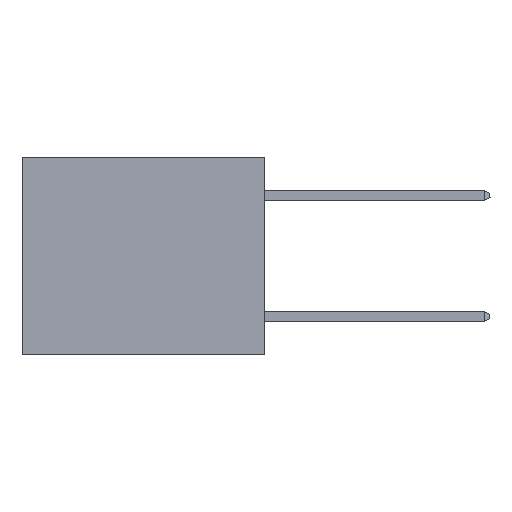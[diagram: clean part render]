
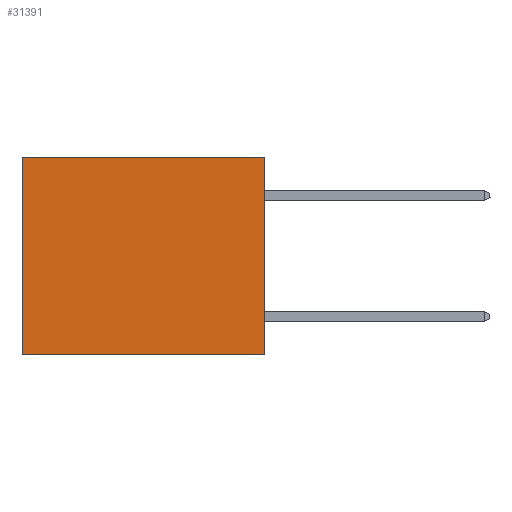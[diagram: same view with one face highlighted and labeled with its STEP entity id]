
A CAD part, left-side view. The second image highlights one B-rep face of the part: STEP entity #31391.
In plain terms, the highlighted planar face has unit normal (-1, 0, 0).
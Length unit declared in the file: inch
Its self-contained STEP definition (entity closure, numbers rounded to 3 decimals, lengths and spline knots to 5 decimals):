
#1313 = LINE ( 'NONE', #6513, #23209 ) ;
#1615 = CARTESIAN_POINT ( 'NONE',  ( 0.3165, 0., -0.49 ) ) ;
#2115 = VERTEX_POINT ( 'NONE', #4589 ) ;
#3891 = ORIENTED_EDGE ( 'NONE', *, *, #5600, .F. ) ;
#4589 = CARTESIAN_POINT ( 'NONE',  ( 0.3165, 0.6, -0.49 ) ) ;
#4840 = EDGE_CURVE ( 'NONE', #29990, #2115, #23736, .T. ) ;
#5600 = EDGE_CURVE ( 'NONE', #15336, #2115, #1313, .T. ) ;
#6211 = DIRECTION ( 'NONE',  ( 0., 0., -1. ) ) ;
#6513 = CARTESIAN_POINT ( 'NONE',  ( 0.3165, 0., -0.49 ) ) ;
#8100 = FACE_OUTER_BOUND ( 'NONE', #31396, .T. ) ;
#8505 = LINE ( 'NONE', #28277, #10466 ) ;
#9212 = DIRECTION ( 'NONE',  ( 0., 1., 0. ) ) ;
#10284 = CARTESIAN_POINT ( 'NONE',  ( 0.3165, 0.6, -0.49 ) ) ;
#10466 = VECTOR ( 'NONE', #6211, 39.37008 ) ;
#10554 = VERTEX_POINT ( 'NONE', #13861 ) ;
#11129 = EDGE_CURVE ( 'NONE', #10554, #29990, #11535, .T. ) ;
#11535 = LINE ( 'NONE', #16831, #26160 ) ;
#12883 = DIRECTION ( 'NONE',  ( 0., 0., -1. ) ) ;
#12912 = ORIENTED_EDGE ( 'NONE', *, *, #11129, .T. ) ;
#13569 = ORIENTED_EDGE ( 'NONE', *, *, #18729, .F. ) ;
#13861 = CARTESIAN_POINT ( 'NONE',  ( 0.3165, 0., 0. ) ) ;
#15336 = VERTEX_POINT ( 'NONE', #22647 ) ;
#16187 = DIRECTION ( 'NONE',  ( 1., 0., 0. ) ) ;
#16831 = CARTESIAN_POINT ( 'NONE',  ( 0.3165, 0., 0. ) ) ;
#18729 = EDGE_CURVE ( 'NONE', #10554, #15336, #8505, .T. ) ;
#19314 = DIRECTION ( 'NONE',  ( 0., 1., 0. ) ) ;
#21388 = VECTOR ( 'NONE', #12883, 39.37008 ) ;
#21995 = CARTESIAN_POINT ( 'NONE',  ( 0.3165, 0.6, 0. ) ) ;
#22647 = CARTESIAN_POINT ( 'NONE',  ( 0.3165, 0., -0.49 ) ) ;
#23209 = VECTOR ( 'NONE', #9212, 39.37008 ) ;
#23736 = LINE ( 'NONE', #10284, #21388 ) ;
#26062 = PLANE ( 'NONE',  #26344 ) ;
#26160 = VECTOR ( 'NONE', #19314, 39.37008 ) ;
#26266 = DIRECTION ( 'NONE',  ( 0., 0., -1. ) ) ;
#26344 = AXIS2_PLACEMENT_3D ( 'NONE', #1615, #16187, #26266 ) ;
#28277 = CARTESIAN_POINT ( 'NONE',  ( 0.3165, 0., -0.49 ) ) ;
#29990 = VERTEX_POINT ( 'NONE', #21995 ) ;
#30311 = ORIENTED_EDGE ( 'NONE', *, *, #4840, .T. ) ;
#31391 = ADVANCED_FACE ( 'NONE', ( #8100 ), #26062, .F. ) ;
#31396 = EDGE_LOOP ( 'NONE', ( #30311, #3891, #13569, #12912 ) ) ;
